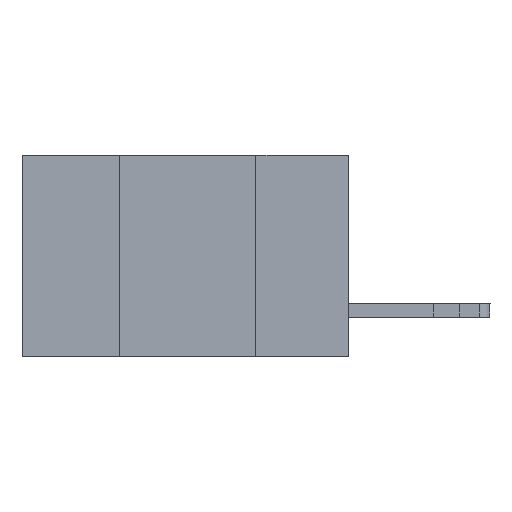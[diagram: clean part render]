
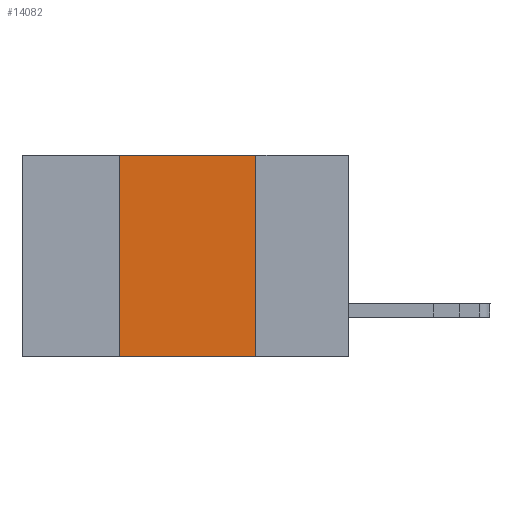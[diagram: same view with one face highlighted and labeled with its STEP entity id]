
A CAD part, left-side view. The second image highlights one B-rep face of the part: STEP entity #14082.
In plain terms, the highlighted planar face has unit normal (-1, 0, 0).
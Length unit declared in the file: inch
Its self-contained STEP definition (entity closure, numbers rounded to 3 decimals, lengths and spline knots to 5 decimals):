
#1619 = EDGE_CURVE ( 'NONE', #3313, #22942, #11623, .T. ) ;
#2332 = LINE ( 'NONE', #13116, #4894 ) ;
#2579 = ORIENTED_EDGE ( 'NONE', *, *, #1619, .F. ) ;
#3107 = ORIENTED_EDGE ( 'NONE', *, *, #9939, .T. ) ;
#3313 = VERTEX_POINT ( 'NONE', #20717 ) ;
#3362 = CARTESIAN_POINT ( 'NONE',  ( 0., 0.6, 0. ) ) ;
#3521 = VECTOR ( 'NONE', #13281, 39.37008 ) ;
#3692 = VERTEX_POINT ( 'NONE', #22897 ) ;
#4139 = DIRECTION ( 'NONE',  ( 0., 0., 1. ) ) ;
#4894 = VECTOR ( 'NONE', #4139, 39.37008 ) ;
#5537 = VECTOR ( 'NONE', #20785, 39.37008 ) ;
#6151 = DIRECTION ( 'NONE',  ( 0., -1., 0. ) ) ;
#6233 = CARTESIAN_POINT ( 'NONE',  ( 0., 0.6, -0.37 ) ) ;
#9939 = EDGE_CURVE ( 'NONE', #22927, #3692, #22923, .T. ) ;
#11585 = CARTESIAN_POINT ( 'NONE',  ( 0., 0.6, 0. ) ) ;
#11623 = LINE ( 'NONE', #11585, #3521 ) ;
#12822 = DIRECTION ( 'NONE',  ( 0., 0., -1. ) ) ;
#13116 = CARTESIAN_POINT ( 'NONE',  ( 0., 0.42, 0. ) ) ;
#13281 = DIRECTION ( 'NONE',  ( 0., -1., 0. ) ) ;
#13363 = LINE ( 'NONE', #19052, #5537 ) ;
#13605 = AXIS2_PLACEMENT_3D ( 'NONE', #3362, #18084, #12822 ) ;
#14018 = ORIENTED_EDGE ( 'NONE', *, *, #17721, .F. ) ;
#14082 = ADVANCED_FACE ( 'NONE', ( #18468 ), #22014, .F. ) ;
#14878 = VECTOR ( 'NONE', #6151, 39.37008 ) ;
#17721 = EDGE_CURVE ( 'NONE', #22942, #3692, #13363, .T. ) ;
#18084 = DIRECTION ( 'NONE',  ( 1., 0., 0. ) ) ;
#18468 = FACE_OUTER_BOUND ( 'NONE', #21297, .T. ) ;
#18936 = EDGE_CURVE ( 'NONE', #22927, #3313, #2332, .T. ) ;
#19052 = CARTESIAN_POINT ( 'NONE',  ( 0., 0.17, 0. ) ) ;
#20717 = CARTESIAN_POINT ( 'NONE',  ( 0., 0.42, 0. ) ) ;
#20785 = DIRECTION ( 'NONE',  ( 0., 0., -1. ) ) ;
#21297 = EDGE_LOOP ( 'NONE', ( #14018, #2579, #22322, #3107 ) ) ;
#22014 = PLANE ( 'NONE',  #13605 ) ;
#22167 = CARTESIAN_POINT ( 'NONE',  ( 0., 0.17, 0. ) ) ;
#22322 = ORIENTED_EDGE ( 'NONE', *, *, #18936, .F. ) ;
#22897 = CARTESIAN_POINT ( 'NONE',  ( 0., 0.17, -0.37 ) ) ;
#22923 = LINE ( 'NONE', #6233, #14878 ) ;
#22927 = VERTEX_POINT ( 'NONE', #23757 ) ;
#22942 = VERTEX_POINT ( 'NONE', #22167 ) ;
#23757 = CARTESIAN_POINT ( 'NONE',  ( 0., 0.42, -0.37 ) ) ;
